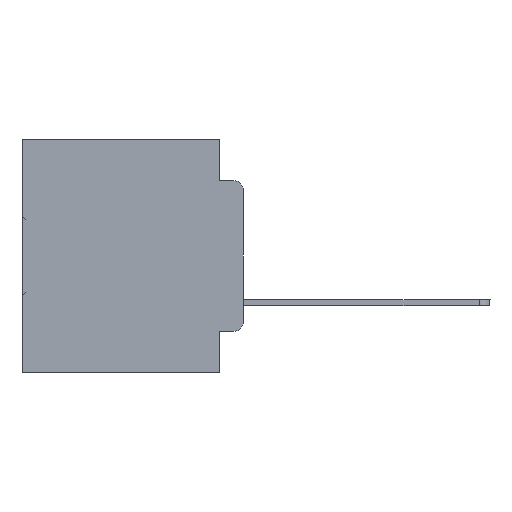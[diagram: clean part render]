
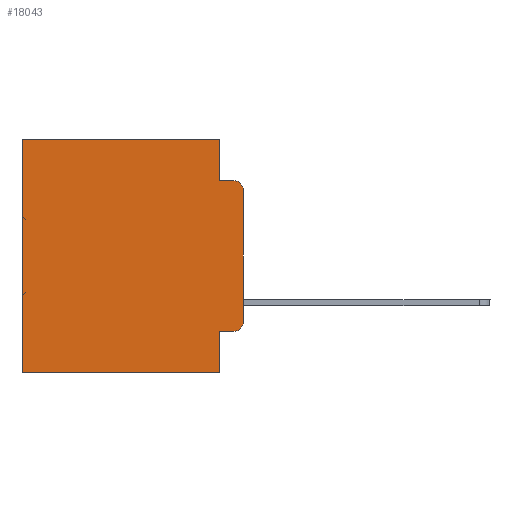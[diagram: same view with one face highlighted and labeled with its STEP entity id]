
A CAD part, left-side view. The second image highlights one B-rep face of the part: STEP entity #18043.
In plain terms, the highlighted planar face has unit normal (-1, 0, 0).
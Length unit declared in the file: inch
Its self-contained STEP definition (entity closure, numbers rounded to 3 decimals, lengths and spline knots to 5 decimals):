
#592 = EDGE_LOOP ( 'NONE', ( #21363, #32354, #2953, #34839, #31697, #34391, #24975, #14449, #23200, #26334 ) ) ;
#1122 = VECTOR ( 'NONE', #27225, 39.37008 ) ;
#2477 = VERTEX_POINT ( 'NONE', #31617 ) ;
#2562 = DIRECTION ( 'NONE',  ( 0., 1., 0. ) ) ;
#2953 = ORIENTED_EDGE ( 'NONE', *, *, #23659, .F. ) ;
#3118 = CIRCLE ( 'NONE', #18024, 0.02 ) ;
#3139 = FACE_OUTER_BOUND ( 'NONE', #592, .T. ) ;
#3415 = CARTESIAN_POINT ( 'NONE',  ( 0.298, 0.473, -0.5 ) ) ;
#3419 = DIRECTION ( 'NONE',  ( 1., 0., 0. ) ) ;
#4580 = VERTEX_POINT ( 'NONE', #7141 ) ;
#4655 = EDGE_CURVE ( 'NONE', #4580, #20070, #13234, .T. ) ;
#5262 = CIRCLE ( 'NONE', #25447, 0.02 ) ;
#6127 = DIRECTION ( 'NONE',  ( 0., 0., -1. ) ) ;
#7012 = LINE ( 'NONE', #24165, #18830 ) ;
#7126 = CARTESIAN_POINT ( 'NONE',  ( 0.298, 0.473, 0. ) ) ;
#7141 = CARTESIAN_POINT ( 'NONE',  ( 0.298, 0.051, -0.5 ) ) ;
#7221 = VERTEX_POINT ( 'NONE', #7627 ) ;
#7241 = VERTEX_POINT ( 'NONE', #21074 ) ;
#7627 = CARTESIAN_POINT ( 'NONE',  ( 0.298, 0.051, -0.4115 ) ) ;
#8295 = LINE ( 'NONE', #33031, #1122 ) ;
#8699 = LINE ( 'NONE', #26817, #26063 ) ;
#9445 = CARTESIAN_POINT ( 'NONE',  ( 0.298, 0., 0. ) ) ;
#9489 = DIRECTION ( 'NONE',  ( -1., 0., 0. ) ) ;
#9801 = VECTOR ( 'NONE', #17578, 39.37008 ) ;
#9854 = CARTESIAN_POINT ( 'NONE',  ( 0.298, 0.02, -0.1085 ) ) ;
#10081 = DIRECTION ( 'NONE',  ( 0., -1., 0. ) ) ;
#10389 = EDGE_CURVE ( 'NONE', #2477, #7241, #26653, .T. ) ;
#11169 = CARTESIAN_POINT ( 'NONE',  ( 0.298, 0.02, -0.0885 ) ) ;
#12064 = EDGE_CURVE ( 'NONE', #7221, #20091, #30379, .T. ) ;
#12410 = CARTESIAN_POINT ( 'NONE',  ( 0.298, 0.051, 0. ) ) ;
#13234 = LINE ( 'NONE', #31673, #20394 ) ;
#14204 = VERTEX_POINT ( 'NONE', #33391 ) ;
#14449 = ORIENTED_EDGE ( 'NONE', *, *, #27948, .F. ) ;
#14734 = EDGE_CURVE ( 'NONE', #25663, #17490, #8295, .T. ) ;
#14857 = CARTESIAN_POINT ( 'NONE',  ( 0.298, 0.02, -0.3915 ) ) ;
#14930 = CARTESIAN_POINT ( 'NONE',  ( 0.298, 0.051, -0.0885 ) ) ;
#15982 = VECTOR ( 'NONE', #28935, 39.37008 ) ;
#16279 = CARTESIAN_POINT ( 'NONE',  ( 0.298, 0.051, -0.4115 ) ) ;
#16841 = CARTESIAN_POINT ( 'NONE',  ( 0.298, 0.02, -0.4115 ) ) ;
#17053 = DIRECTION ( 'NONE',  ( -1., 0., 0. ) ) ;
#17490 = VERTEX_POINT ( 'NONE', #33784 ) ;
#17578 = DIRECTION ( 'NONE',  ( 0., 0., -1. ) ) ;
#18024 = AXIS2_PLACEMENT_3D ( 'NONE', #9854, #9489, #28686 ) ;
#18043 = ADVANCED_FACE ( 'NONE', ( #3139 ), #22650, .F. ) ;
#18562 = EDGE_CURVE ( 'NONE', #20091, #7241, #5262, .T. ) ;
#18830 = VECTOR ( 'NONE', #24275, 39.37008 ) ;
#19036 = DIRECTION ( 'NONE',  ( 0., -1., 0. ) ) ;
#19597 = CARTESIAN_POINT ( 'NONE',  ( 0.298, 0., 0. ) ) ;
#20070 = VERTEX_POINT ( 'NONE', #3415 ) ;
#20091 = VERTEX_POINT ( 'NONE', #16841 ) ;
#20394 = VECTOR ( 'NONE', #23756, 39.37008 ) ;
#21074 = CARTESIAN_POINT ( 'NONE',  ( 0.298, 0., -0.3915 ) ) ;
#21363 = ORIENTED_EDGE ( 'NONE', *, *, #10389, .F. ) ;
#22302 = LINE ( 'NONE', #7126, #15982 ) ;
#22650 = PLANE ( 'NONE',  #31810 ) ;
#23200 = ORIENTED_EDGE ( 'NONE', *, *, #12064, .T. ) ;
#23659 = EDGE_CURVE ( 'NONE', #17490, #26302, #29362, .T. ) ;
#23756 = DIRECTION ( 'NONE',  ( 0., 1., 0. ) ) ;
#24165 = CARTESIAN_POINT ( 'NONE',  ( 0.298, 0.051, 0. ) ) ;
#24275 = DIRECTION ( 'NONE',  ( 0., 0., -1. ) ) ;
#24975 = ORIENTED_EDGE ( 'NONE', *, *, #4655, .F. ) ;
#25447 = AXIS2_PLACEMENT_3D ( 'NONE', #14857, #17053, #30880 ) ;
#25663 = VERTEX_POINT ( 'NONE', #12410 ) ;
#26063 = VECTOR ( 'NONE', #2562, 39.37008 ) ;
#26302 = VERTEX_POINT ( 'NONE', #11169 ) ;
#26334 = ORIENTED_EDGE ( 'NONE', *, *, #18562, .T. ) ;
#26486 = EDGE_CURVE ( 'NONE', #14204, #20070, #22302, .T. ) ;
#26653 = LINE ( 'NONE', #9445, #9801 ) ;
#26817 = CARTESIAN_POINT ( 'NONE',  ( 0.298, 0., 0. ) ) ;
#27225 = DIRECTION ( 'NONE',  ( 0., 0., -1. ) ) ;
#27948 = EDGE_CURVE ( 'NONE', #7221, #4580, #7012, .T. ) ;
#28087 = VECTOR ( 'NONE', #10081, 39.37008 ) ;
#28686 = DIRECTION ( 'NONE',  ( 0., 0., -1. ) ) ;
#28924 = EDGE_CURVE ( 'NONE', #2477, #26302, #3118, .T. ) ;
#28935 = DIRECTION ( 'NONE',  ( 0., 0., -1. ) ) ;
#29362 = LINE ( 'NONE', #14930, #28087 ) ;
#30379 = LINE ( 'NONE', #16279, #32913 ) ;
#30880 = DIRECTION ( 'NONE',  ( 0., 0., -1. ) ) ;
#31617 = CARTESIAN_POINT ( 'NONE',  ( 0.298, 0., -0.1085 ) ) ;
#31673 = CARTESIAN_POINT ( 'NONE',  ( 0.298, 0., -0.5 ) ) ;
#31697 = ORIENTED_EDGE ( 'NONE', *, *, #31783, .T. ) ;
#31783 = EDGE_CURVE ( 'NONE', #25663, #14204, #8699, .T. ) ;
#31810 = AXIS2_PLACEMENT_3D ( 'NONE', #19597, #3419, #6127 ) ;
#32354 = ORIENTED_EDGE ( 'NONE', *, *, #28924, .T. ) ;
#32913 = VECTOR ( 'NONE', #19036, 39.37008 ) ;
#33031 = CARTESIAN_POINT ( 'NONE',  ( 0.298, 0.051, 0. ) ) ;
#33391 = CARTESIAN_POINT ( 'NONE',  ( 0.298, 0.473, 0. ) ) ;
#33784 = CARTESIAN_POINT ( 'NONE',  ( 0.298, 0.051, -0.0885 ) ) ;
#34391 = ORIENTED_EDGE ( 'NONE', *, *, #26486, .T. ) ;
#34839 = ORIENTED_EDGE ( 'NONE', *, *, #14734, .F. ) ;
